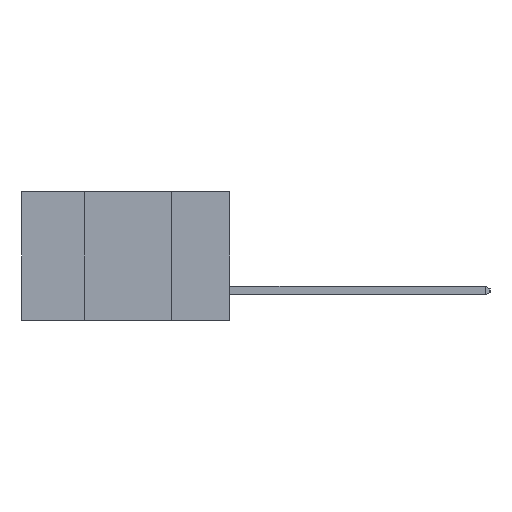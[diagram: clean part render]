
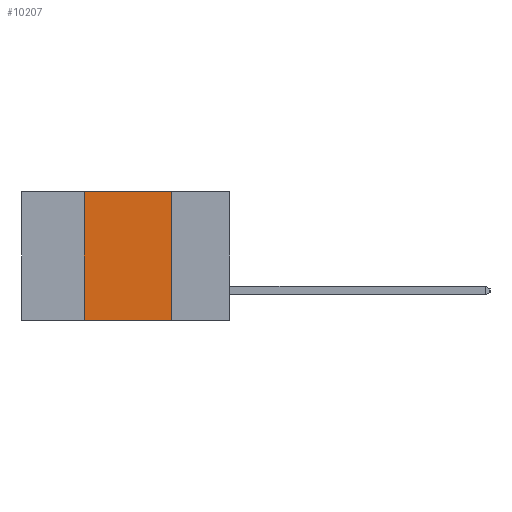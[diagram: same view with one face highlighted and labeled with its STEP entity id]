
A CAD part, left-side view. The second image highlights one B-rep face of the part: STEP entity #10207.
In plain terms, the highlighted planar face has unit normal (-1, 0, 0).
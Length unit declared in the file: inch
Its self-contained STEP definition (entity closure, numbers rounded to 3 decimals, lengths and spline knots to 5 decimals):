
#409 = ORIENTED_EDGE ( 'NONE', *, *, #5965, .T. ) ;
#511 = LINE ( 'NONE', #12851, #3062 ) ;
#870 = EDGE_CURVE ( 'NONE', #8273, #9049, #511, .T. ) ;
#1501 = CARTESIAN_POINT ( 'NONE',  ( 0., 0.42, -0.37 ) ) ;
#2570 = VECTOR ( 'NONE', #13488, 39.37008 ) ;
#2673 = EDGE_LOOP ( 'NONE', ( #14264, #10398, #4292, #409 ) ) ;
#3044 = VECTOR ( 'NONE', #3055, 39.37008 ) ;
#3055 = DIRECTION ( 'NONE',  ( 0., -1., 0. ) ) ;
#3062 = VECTOR ( 'NONE', #12873, 39.37008 ) ;
#3500 = CARTESIAN_POINT ( 'NONE',  ( 0., 0.17, -0.37 ) ) ;
#4246 = EDGE_CURVE ( 'NONE', #9049, #6657, #6024, .T. ) ;
#4292 = ORIENTED_EDGE ( 'NONE', *, *, #870, .F. ) ;
#4303 = CARTESIAN_POINT ( 'NONE',  ( 0., 0.6, 0. ) ) ;
#5591 = DIRECTION ( 'NONE',  ( 0., 0., -1. ) ) ;
#5935 = CARTESIAN_POINT ( 'NONE',  ( 0., 0.17, -0.37 ) ) ;
#5965 = EDGE_CURVE ( 'NONE', #8273, #7331, #9298, .T. ) ;
#5994 = CARTESIAN_POINT ( 'NONE',  ( 0., 0.6, -0.37 ) ) ;
#6024 = LINE ( 'NONE', #10594, #3044 ) ;
#6526 = VECTOR ( 'NONE', #10890, 39.37008 ) ;
#6657 = VERTEX_POINT ( 'NONE', #8605 ) ;
#7331 = VERTEX_POINT ( 'NONE', #3500 ) ;
#8273 = VERTEX_POINT ( 'NONE', #1501 ) ;
#8605 = CARTESIAN_POINT ( 'NONE',  ( 0., 0.17, 0. ) ) ;
#8717 = AXIS2_PLACEMENT_3D ( 'NONE', #4303, #13108, #5591 ) ;
#9049 = VERTEX_POINT ( 'NONE', #9364 ) ;
#9298 = LINE ( 'NONE', #5994, #2570 ) ;
#9334 = PLANE ( 'NONE',  #8717 ) ;
#9364 = CARTESIAN_POINT ( 'NONE',  ( 0., 0.42, 0. ) ) ;
#9856 = LINE ( 'NONE', #5935, #6526 ) ;
#10207 = ADVANCED_FACE ( 'NONE', ( #13772 ), #9334, .F. ) ;
#10398 = ORIENTED_EDGE ( 'NONE', *, *, #4246, .F. ) ;
#10594 = CARTESIAN_POINT ( 'NONE',  ( 0., 0.6, 0. ) ) ;
#10890 = DIRECTION ( 'NONE',  ( 0., 0., -1. ) ) ;
#11299 = EDGE_CURVE ( 'NONE', #6657, #7331, #9856, .T. ) ;
#12851 = CARTESIAN_POINT ( 'NONE',  ( 0., 0.42, -0.37 ) ) ;
#12873 = DIRECTION ( 'NONE',  ( 0., 0., 1. ) ) ;
#13108 = DIRECTION ( 'NONE',  ( 1., 0., 0. ) ) ;
#13488 = DIRECTION ( 'NONE',  ( 0., -1., 0. ) ) ;
#13772 = FACE_OUTER_BOUND ( 'NONE', #2673, .T. ) ;
#14264 = ORIENTED_EDGE ( 'NONE', *, *, #11299, .F. ) ;
